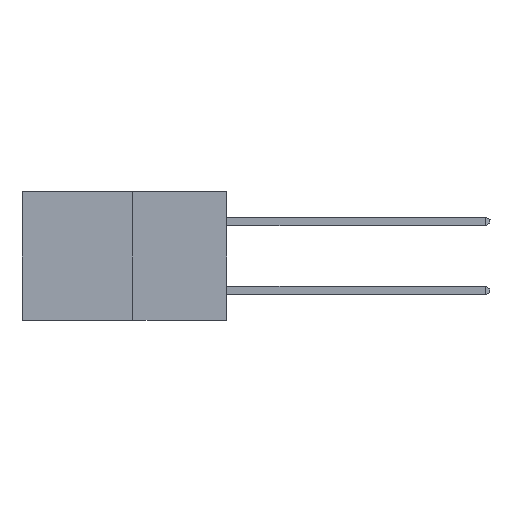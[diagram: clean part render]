
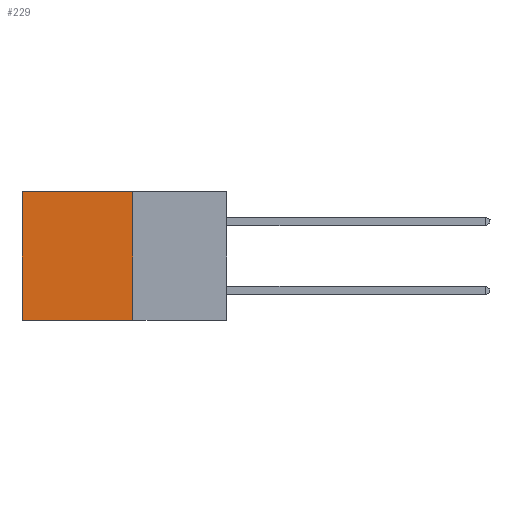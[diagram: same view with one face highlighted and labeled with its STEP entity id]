
A CAD part, left-side view. The second image highlights one B-rep face of the part: STEP entity #229.
In plain terms, the highlighted planar face has unit normal (-1, 0, 0).
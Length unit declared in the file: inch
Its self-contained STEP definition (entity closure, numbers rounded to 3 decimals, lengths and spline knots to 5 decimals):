
#132 = VECTOR ( 'NONE', #16807, 39.37008 ) ;
#229 = ADVANCED_FACE ( 'NONE', ( #15161 ), #7547, .F. ) ;
#1508 = DIRECTION ( 'NONE',  ( 0., 0., -1. ) ) ;
#1681 = EDGE_CURVE ( 'NONE', #18448, #12117, #4457, .T. ) ;
#2356 = VECTOR ( 'NONE', #6451, 39.37008 ) ;
#3191 = VERTEX_POINT ( 'NONE', #11139 ) ;
#4457 = LINE ( 'NONE', #6639, #132 ) ;
#5072 = VECTOR ( 'NONE', #1508, 39.37008 ) ;
#5659 = LINE ( 'NONE', #23000, #5072 ) ;
#6451 = DIRECTION ( 'NONE',  ( 0., 0., -1. ) ) ;
#6639 = CARTESIAN_POINT ( 'NONE',  ( 0.277, 0.27, -0.37 ) ) ;
#6940 = ORIENTED_EDGE ( 'NONE', *, *, #1681, .F. ) ;
#7547 = PLANE ( 'NONE',  #10629 ) ;
#8160 = CARTESIAN_POINT ( 'NONE',  ( 0.277, 0.27, -0.37 ) ) ;
#8940 = CARTESIAN_POINT ( 'NONE',  ( 0.277, 0.27, -0.37 ) ) ;
#10629 = AXIS2_PLACEMENT_3D ( 'NONE', #8940, #15057, #15103 ) ;
#10962 = EDGE_CURVE ( 'NONE', #21485, #18448, #12497, .T. ) ;
#11139 = CARTESIAN_POINT ( 'NONE',  ( 0.277, 0.59, 0. ) ) ;
#12117 = VERTEX_POINT ( 'NONE', #18334 ) ;
#12497 = LINE ( 'NONE', #8160, #2356 ) ;
#13767 = EDGE_CURVE ( 'NONE', #21485, #3191, #23238, .T. ) ;
#15057 = DIRECTION ( 'NONE',  ( 1., 0., 0. ) ) ;
#15103 = DIRECTION ( 'NONE',  ( 0., 0., -1. ) ) ;
#15161 = FACE_OUTER_BOUND ( 'NONE', #22119, .T. ) ;
#15602 = CARTESIAN_POINT ( 'NONE',  ( 0.277, 0.27, -0.37 ) ) ;
#16807 = DIRECTION ( 'NONE',  ( 0., 1., 0. ) ) ;
#17472 = CARTESIAN_POINT ( 'NONE',  ( 0.277, 0.27, 0. ) ) ;
#18334 = CARTESIAN_POINT ( 'NONE',  ( 0.277, 0.59, -0.37 ) ) ;
#18448 = VERTEX_POINT ( 'NONE', #15602 ) ;
#19349 = CARTESIAN_POINT ( 'NONE',  ( 0.277, 0.27, 0. ) ) ;
#19674 = VECTOR ( 'NONE', #22768, 39.37008 ) ;
#19757 = ORIENTED_EDGE ( 'NONE', *, *, #20796, .T. ) ;
#20338 = ORIENTED_EDGE ( 'NONE', *, *, #10962, .F. ) ;
#20796 = EDGE_CURVE ( 'NONE', #3191, #12117, #5659, .T. ) ;
#21360 = ORIENTED_EDGE ( 'NONE', *, *, #13767, .T. ) ;
#21485 = VERTEX_POINT ( 'NONE', #19349 ) ;
#22119 = EDGE_LOOP ( 'NONE', ( #19757, #6940, #20338, #21360 ) ) ;
#22768 = DIRECTION ( 'NONE',  ( 0., 1., 0. ) ) ;
#23000 = CARTESIAN_POINT ( 'NONE',  ( 0.277, 0.59, -0.37 ) ) ;
#23238 = LINE ( 'NONE', #17472, #19674 ) ;
